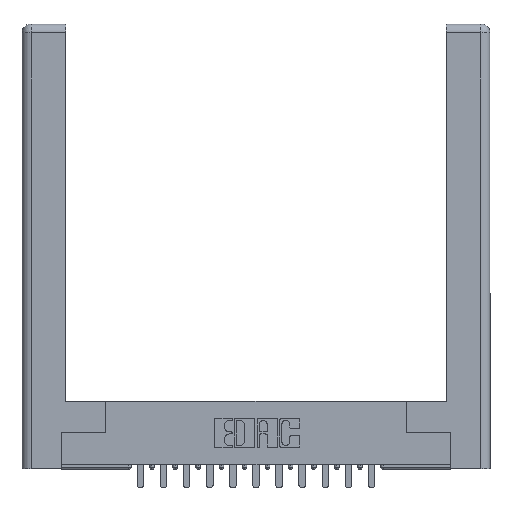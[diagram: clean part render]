
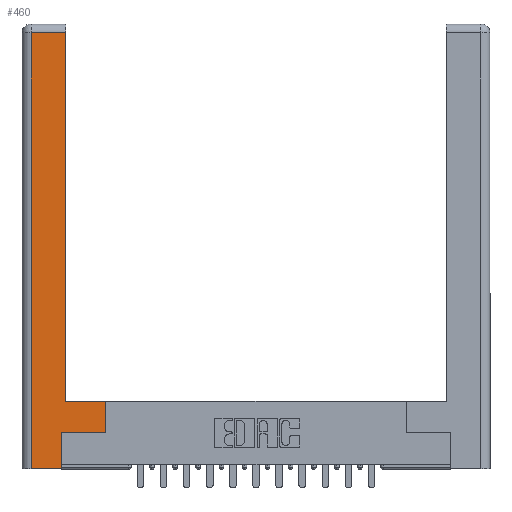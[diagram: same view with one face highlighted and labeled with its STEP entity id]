
A CAD part, top view. The second image highlights one B-rep face of the part: STEP entity #460.
In plain terms, the highlighted planar face has unit normal (0, 0, 1).
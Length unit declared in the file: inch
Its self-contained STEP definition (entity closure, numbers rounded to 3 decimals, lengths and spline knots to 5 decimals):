
#455 = CARTESIAN_POINT ( 'NONE',  ( 0.0615, 0., 0. ) ) ;
#460 = ADVANCED_FACE ( 'NONE', ( #4605 ), #3788, .F. ) ;
#759 = DIRECTION ( 'NONE',  ( 0., 1., 0. ) ) ;
#1029 = LINE ( 'NONE', #1283, #8453 ) ;
#1071 = DIRECTION ( 'NONE',  ( 0., 1., 0. ) ) ;
#1283 = CARTESIAN_POINT ( 'NONE',  ( 0.295, 3., 0. ) ) ;
#1439 = LINE ( 'NONE', #15171, #8884 ) ;
#2146 = LINE ( 'NONE', #7427, #14044 ) ;
#2397 = EDGE_CURVE ( 'NONE', #11419, #9945, #14717, .T. ) ;
#2738 = ORIENTED_EDGE ( 'NONE', *, *, #8797, .T. ) ;
#2970 = EDGE_CURVE ( 'NONE', #9475, #11419, #17130, .T. ) ;
#3170 = ORIENTED_EDGE ( 'NONE', *, *, #3653, .T. ) ;
#3570 = ORIENTED_EDGE ( 'NONE', *, *, #8194, .T. ) ;
#3617 = ORIENTED_EDGE ( 'NONE', *, *, #6196, .T. ) ;
#3653 = EDGE_CURVE ( 'NONE', #8767, #4025, #1029, .T. ) ;
#3783 = DIRECTION ( 'NONE',  ( 0., 1., 0. ) ) ;
#3788 = PLANE ( 'NONE',  #9897 ) ;
#4025 = VERTEX_POINT ( 'NONE', #7792 ) ;
#4347 = CARTESIAN_POINT ( 'NONE',  ( 0.265, 0.245, 0. ) ) ;
#4605 = FACE_OUTER_BOUND ( 'NONE', #11634, .T. ) ;
#5611 = LINE ( 'NONE', #9949, #8257 ) ;
#6196 = EDGE_CURVE ( 'NONE', #12075, #6689, #10545, .T. ) ;
#6557 = VERTEX_POINT ( 'NONE', #7068 ) ;
#6689 = VERTEX_POINT ( 'NONE', #17386 ) ;
#6951 = DIRECTION ( 'NONE',  ( 1., 0., 0. ) ) ;
#7068 = CARTESIAN_POINT ( 'NONE',  ( 0.0615, 2.94, 0. ) ) ;
#7427 = CARTESIAN_POINT ( 'NONE',  ( 0.0615, 0., 0. ) ) ;
#7792 = CARTESIAN_POINT ( 'NONE',  ( 0.295, 2.94, 0. ) ) ;
#7950 = DIRECTION ( 'NONE',  ( -1., 0., 0. ) ) ;
#8011 = DIRECTION ( 'NONE',  ( 0., 0., -1. ) ) ;
#8194 = EDGE_CURVE ( 'NONE', #6557, #9475, #2146, .T. ) ;
#8257 = VECTOR ( 'NONE', #8580, 39.37008 ) ;
#8453 = VECTOR ( 'NONE', #3783, 39.37008 ) ;
#8580 = DIRECTION ( 'NONE',  ( -1., 0., 0. ) ) ;
#8767 = VERTEX_POINT ( 'NONE', #17066 ) ;
#8797 = EDGE_CURVE ( 'NONE', #4025, #6557, #5611, .T. ) ;
#8884 = VECTOR ( 'NONE', #15740, 39.37008 ) ;
#9475 = VERTEX_POINT ( 'NONE', #455 ) ;
#9605 = CARTESIAN_POINT ( 'NONE',  ( 0.265, 0., 0. ) ) ;
#9897 = AXIS2_PLACEMENT_3D ( 'NONE', #10725, #8011, #7950 ) ;
#9912 = EDGE_CURVE ( 'NONE', #9945, #12075, #1439, .T. ) ;
#9945 = VERTEX_POINT ( 'NONE', #17101 ) ;
#9949 = CARTESIAN_POINT ( 'NONE',  ( 0.0615, 2.94, 0. ) ) ;
#10316 = ORIENTED_EDGE ( 'NONE', *, *, #2397, .T. ) ;
#10491 = ORIENTED_EDGE ( 'NONE', *, *, #9912, .T. ) ;
#10545 = LINE ( 'NONE', #13152, #10981 ) ;
#10725 = CARTESIAN_POINT ( 'NONE',  ( 0., 0., 0. ) ) ;
#10853 = ORIENTED_EDGE ( 'NONE', *, *, #16557, .T. ) ;
#10981 = VECTOR ( 'NONE', #759, 39.37008 ) ;
#11419 = VERTEX_POINT ( 'NONE', #14970 ) ;
#11634 = EDGE_LOOP ( 'NONE', ( #3170, #2738, #3570, #16257, #10316, #10491, #3617, #10853 ) ) ;
#12071 = VECTOR ( 'NONE', #1071, 39.37008 ) ;
#12075 = VERTEX_POINT ( 'NONE', #14517 ) ;
#12603 = DIRECTION ( 'NONE',  ( -1., 0., 0. ) ) ;
#13152 = CARTESIAN_POINT ( 'NONE',  ( 0.565, 0.45, 0. ) ) ;
#14044 = VECTOR ( 'NONE', #15903, 39.37008 ) ;
#14517 = CARTESIAN_POINT ( 'NONE',  ( 0.565, 0.245, 0. ) ) ;
#14717 = LINE ( 'NONE', #4347, #12071 ) ;
#14911 = VECTOR ( 'NONE', #6951, 39.37008 ) ;
#14970 = CARTESIAN_POINT ( 'NONE',  ( 0.265, 0., 0. ) ) ;
#15171 = CARTESIAN_POINT ( 'NONE',  ( 0.565, 0.245, 0. ) ) ;
#15182 = VECTOR ( 'NONE', #12603, 39.37008 ) ;
#15740 = DIRECTION ( 'NONE',  ( 1., 0., 0. ) ) ;
#15903 = DIRECTION ( 'NONE',  ( 0., -1., 0. ) ) ;
#16257 = ORIENTED_EDGE ( 'NONE', *, *, #2970, .T. ) ;
#16557 = EDGE_CURVE ( 'NONE', #6689, #8767, #17831, .T. ) ;
#17038 = CARTESIAN_POINT ( 'NONE',  ( 0.295, 0.45, 0. ) ) ;
#17066 = CARTESIAN_POINT ( 'NONE',  ( 0.295, 0.45, 0. ) ) ;
#17101 = CARTESIAN_POINT ( 'NONE',  ( 0.265, 0.245, 0. ) ) ;
#17130 = LINE ( 'NONE', #9605, #14911 ) ;
#17386 = CARTESIAN_POINT ( 'NONE',  ( 0.565, 0.45, 0. ) ) ;
#17831 = LINE ( 'NONE', #17038, #15182 ) ;
